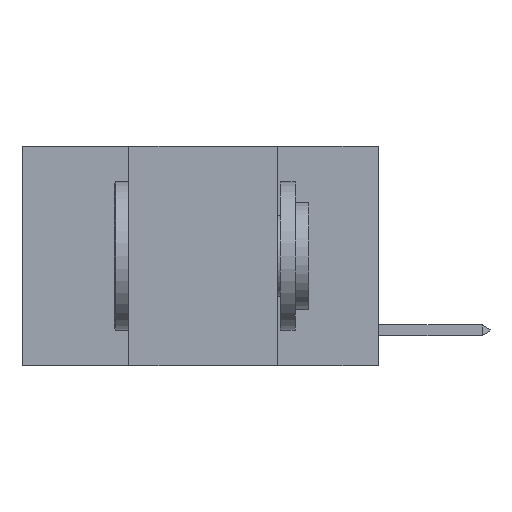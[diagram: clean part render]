
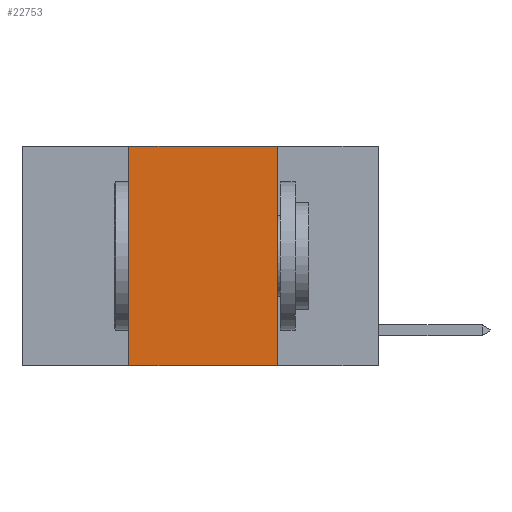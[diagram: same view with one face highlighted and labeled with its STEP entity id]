
A CAD part, left-side view. The second image highlights one B-rep face of the part: STEP entity #22753.
In plain terms, the highlighted planar face has unit normal (-1, 0, 0).
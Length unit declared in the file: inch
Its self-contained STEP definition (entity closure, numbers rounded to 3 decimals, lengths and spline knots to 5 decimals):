
#1979 = EDGE_CURVE ( 'NONE', #12997, #27417, #9366, .T. ) ;
#1981 = CARTESIAN_POINT ( 'NONE',  ( 0., 0.17, 0. ) ) ;
#2663 = ORIENTED_EDGE ( 'NONE', *, *, #1979, .T. ) ;
#4322 = FACE_OUTER_BOUND ( 'NONE', #17173, .T. ) ;
#4937 = DIRECTION ( 'NONE',  ( 0., 0., 1. ) ) ;
#5524 = EDGE_CURVE ( 'NONE', #8607, #27417, #8850, .T. ) ;
#5921 = DIRECTION ( 'NONE',  ( 0., 0., -1. ) ) ;
#6183 = VERTEX_POINT ( 'NONE', #24575 ) ;
#6595 = VECTOR ( 'NONE', #4937, 39.37008 ) ;
#7264 = VECTOR ( 'NONE', #20286, 39.37008 ) ;
#8079 = CARTESIAN_POINT ( 'NONE',  ( 0., 0.17, -0.37 ) ) ;
#8149 = VECTOR ( 'NONE', #10709, 39.37008 ) ;
#8607 = VERTEX_POINT ( 'NONE', #19926 ) ;
#8850 = LINE ( 'NONE', #1981, #8149 ) ;
#9366 = LINE ( 'NONE', #26797, #7264 ) ;
#9414 = ORIENTED_EDGE ( 'NONE', *, *, #15870, .F. ) ;
#10709 = DIRECTION ( 'NONE',  ( 0., 0., -1. ) ) ;
#12997 = VERTEX_POINT ( 'NONE', #13815 ) ;
#13492 = LINE ( 'NONE', #18093, #6595 ) ;
#13815 = CARTESIAN_POINT ( 'NONE',  ( 0., 0.42, -0.37 ) ) ;
#14498 = DIRECTION ( 'NONE',  ( 1., 0., 0. ) ) ;
#15870 = EDGE_CURVE ( 'NONE', #12997, #6183, #13492, .T. ) ;
#16039 = CARTESIAN_POINT ( 'NONE',  ( 0., 0.6, 0. ) ) ;
#16945 = PLANE ( 'NONE',  #24152 ) ;
#17173 = EDGE_LOOP ( 'NONE', ( #19740, #18229, #9414, #2663 ) ) ;
#18093 = CARTESIAN_POINT ( 'NONE',  ( 0., 0.42, 0. ) ) ;
#18229 = ORIENTED_EDGE ( 'NONE', *, *, #19370, .F. ) ;
#18943 = CARTESIAN_POINT ( 'NONE',  ( 0., 0.6, 0. ) ) ;
#19370 = EDGE_CURVE ( 'NONE', #6183, #8607, #22987, .T. ) ;
#19740 = ORIENTED_EDGE ( 'NONE', *, *, #5524, .F. ) ;
#19926 = CARTESIAN_POINT ( 'NONE',  ( 0., 0.17, 0. ) ) ;
#20286 = DIRECTION ( 'NONE',  ( 0., -1., 0. ) ) ;
#22753 = ADVANCED_FACE ( 'NONE', ( #4322 ), #16945, .F. ) ;
#22987 = LINE ( 'NONE', #16039, #25071 ) ;
#24152 = AXIS2_PLACEMENT_3D ( 'NONE', #18943, #14498, #5921 ) ;
#24575 = CARTESIAN_POINT ( 'NONE',  ( 0., 0.42, 0. ) ) ;
#25071 = VECTOR ( 'NONE', #25091, 39.37008 ) ;
#25091 = DIRECTION ( 'NONE',  ( 0., -1., 0. ) ) ;
#26797 = CARTESIAN_POINT ( 'NONE',  ( 0., 0.6, -0.37 ) ) ;
#27417 = VERTEX_POINT ( 'NONE', #8079 ) ;
